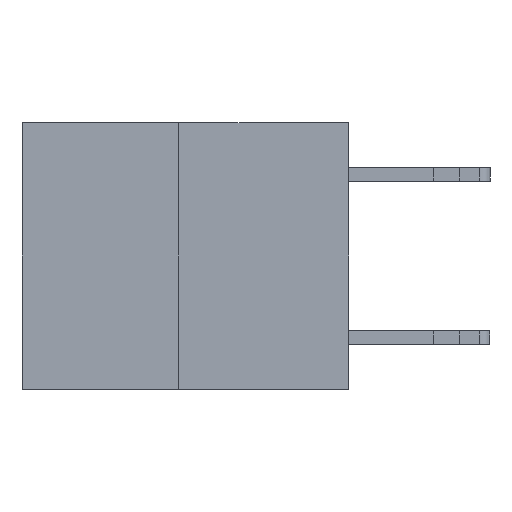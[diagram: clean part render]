
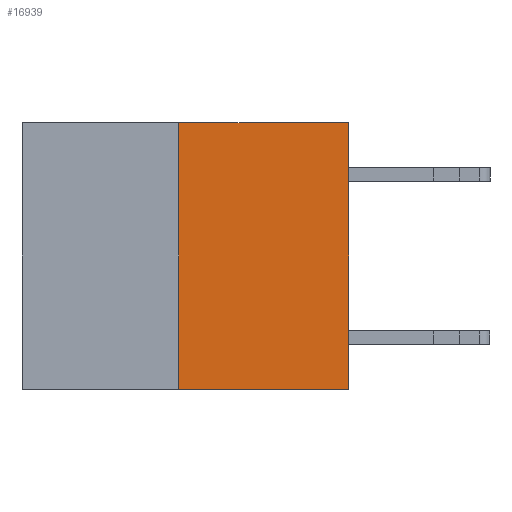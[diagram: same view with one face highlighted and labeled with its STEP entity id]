
A CAD part, left-side view. The second image highlights one B-rep face of the part: STEP entity #16939.
In plain terms, the highlighted planar face has unit normal (-1, 0, 0).
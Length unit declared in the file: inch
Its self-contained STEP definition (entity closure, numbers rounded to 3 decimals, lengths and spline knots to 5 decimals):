
#191 = LINE ( 'NONE', #14417, #14028 ) ;
#616 = DIRECTION ( 'NONE',  ( 0., -1., 0. ) ) ;
#921 = ORIENTED_EDGE ( 'NONE', *, *, #1254, .F. ) ;
#1254 = EDGE_CURVE ( 'NONE', #9954, #14813, #2681, .T. ) ;
#2333 = CARTESIAN_POINT ( 'NONE',  ( 0., 0.6, 0. ) ) ;
#2532 = ORIENTED_EDGE ( 'NONE', *, *, #8812, .T. ) ;
#2645 = DIRECTION ( 'NONE',  ( 0., 0., 1. ) ) ;
#2681 = LINE ( 'NONE', #2333, #16505 ) ;
#3193 = AXIS2_PLACEMENT_3D ( 'NONE', #5758, #16679, #15404 ) ;
#3221 = EDGE_CURVE ( 'NONE', #10343, #9954, #11898, .T. ) ;
#3462 = CARTESIAN_POINT ( 'NONE',  ( 0., 0.312, -0.49 ) ) ;
#4376 = EDGE_CURVE ( 'NONE', #17366, #14813, #191, .T. ) ;
#5368 = DIRECTION ( 'NONE',  ( 0., -1., 0. ) ) ;
#5758 = CARTESIAN_POINT ( 'NONE',  ( 0., 0.6, 0. ) ) ;
#7543 = DIRECTION ( 'NONE',  ( 0., 0., 1. ) ) ;
#7959 = CARTESIAN_POINT ( 'NONE',  ( 0., 0.312, 0. ) ) ;
#8049 = CARTESIAN_POINT ( 'NONE',  ( 0., 0.312, -0.49 ) ) ;
#8725 = EDGE_LOOP ( 'NONE', ( #10301, #2532, #9181, #921 ) ) ;
#8812 = EDGE_CURVE ( 'NONE', #10343, #17366, #15685, .T. ) ;
#9181 = ORIENTED_EDGE ( 'NONE', *, *, #4376, .T. ) ;
#9298 = CARTESIAN_POINT ( 'NONE',  ( 0., 0., 0. ) ) ;
#9954 = VERTEX_POINT ( 'NONE', #7959 ) ;
#10301 = ORIENTED_EDGE ( 'NONE', *, *, #3221, .F. ) ;
#10343 = VERTEX_POINT ( 'NONE', #3462 ) ;
#11828 = VECTOR ( 'NONE', #5368, 39.37008 ) ;
#11898 = LINE ( 'NONE', #8049, #13183 ) ;
#11907 = CARTESIAN_POINT ( 'NONE',  ( 0., 0., -0.49 ) ) ;
#13183 = VECTOR ( 'NONE', #2645, 39.37008 ) ;
#13515 = CARTESIAN_POINT ( 'NONE',  ( 0., 0.6, -0.49 ) ) ;
#13919 = PLANE ( 'NONE',  #3193 ) ;
#14028 = VECTOR ( 'NONE', #7543, 39.37008 ) ;
#14417 = CARTESIAN_POINT ( 'NONE',  ( 0., 0., 0. ) ) ;
#14813 = VERTEX_POINT ( 'NONE', #9298 ) ;
#15404 = DIRECTION ( 'NONE',  ( 0., 0., -1. ) ) ;
#15527 = FACE_OUTER_BOUND ( 'NONE', #8725, .T. ) ;
#15685 = LINE ( 'NONE', #13515, #11828 ) ;
#16505 = VECTOR ( 'NONE', #616, 39.37008 ) ;
#16679 = DIRECTION ( 'NONE',  ( 1., 0., 0. ) ) ;
#16939 = ADVANCED_FACE ( 'NONE', ( #15527 ), #13919, .F. ) ;
#17366 = VERTEX_POINT ( 'NONE', #11907 ) ;
